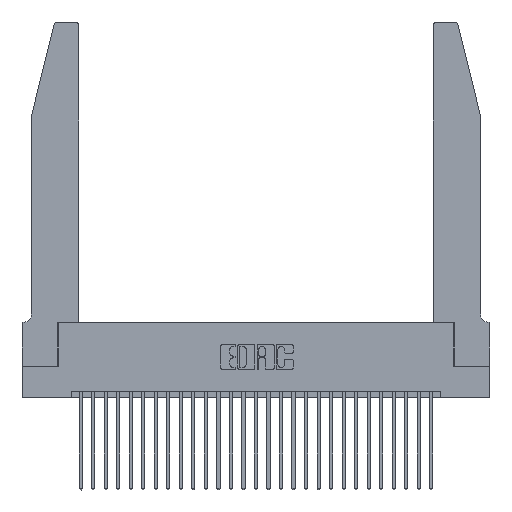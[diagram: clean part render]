
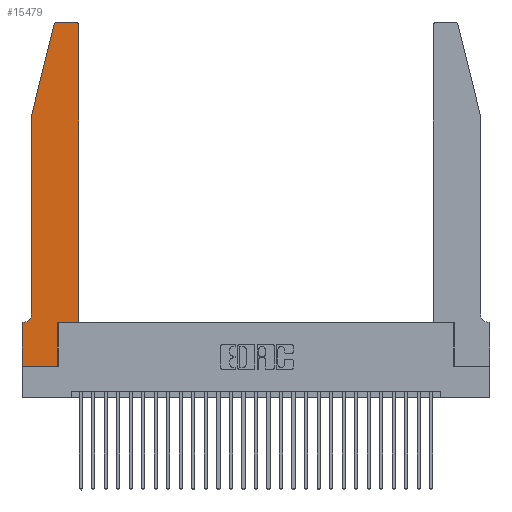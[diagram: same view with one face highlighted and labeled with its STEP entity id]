
A CAD part, top view. The second image highlights one B-rep face of the part: STEP entity #15479.
In plain terms, the highlighted planar face has unit normal (0, 0, 1).
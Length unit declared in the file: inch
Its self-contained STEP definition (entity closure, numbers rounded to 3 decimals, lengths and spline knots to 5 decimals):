
#150 = EDGE_CURVE ( 'NONE', #22027, #7102, #5964, .T. ) ;
#335 = CARTESIAN_POINT ( 'NONE',  ( 0.4505, 0.35, 0.37 ) ) ;
#549 = LINE ( 'NONE', #19431, #22512 ) ;
#706 = EDGE_CURVE ( 'NONE', #18985, #27668, #26886, .T. ) ;
#952 = ORIENTED_EDGE ( 'NONE', *, *, #706, .T. ) ;
#983 = ORIENTED_EDGE ( 'NONE', *, *, #17889, .T. ) ;
#1595 = VECTOR ( 'NONE', #10369, 39.37008 ) ;
#1600 = DIRECTION ( 'NONE',  ( 0., 0., 1. ) ) ;
#2315 = VERTEX_POINT ( 'NONE', #2986 ) ;
#2401 = EDGE_CURVE ( 'NONE', #27358, #15145, #27176, .T. ) ;
#2516 = FACE_OUTER_BOUND ( 'NONE', #24900, .T. ) ;
#2548 = DIRECTION ( 'NONE',  ( 1., 0., 0. ) ) ;
#2813 = CARTESIAN_POINT ( 'NONE',  ( 0.0055, 0.42, 0.37 ) ) ;
#2986 = CARTESIAN_POINT ( 'NONE',  ( 0.0055, 0.35, 0.37 ) ) ;
#3007 = LINE ( 'NONE', #5709, #1595 ) ;
#3257 = LINE ( 'NONE', #4641, #13493 ) ;
#3442 = CARTESIAN_POINT ( 'NONE',  ( 0.4205, 2.75, 0.37 ) ) ;
#4108 = CARTESIAN_POINT ( 'NONE',  ( 0.0755, 2., 0.37 ) ) ;
#4473 = VECTOR ( 'NONE', #17967, 39.37008 ) ;
#4641 = CARTESIAN_POINT ( 'NONE',  ( 0.2865, 0.35, 0.37 ) ) ;
#4757 = AXIS2_PLACEMENT_3D ( 'NONE', #26374, #1600, #26477 ) ;
#5021 = LINE ( 'NONE', #335, #22012 ) ;
#5185 = ORIENTED_EDGE ( 'NONE', *, *, #150, .T. ) ;
#5709 = CARTESIAN_POINT ( 'NONE',  ( 0.2605, 2.75, 0.37 ) ) ;
#5964 = LINE ( 'NONE', #22338, #27705 ) ;
#6318 = CARTESIAN_POINT ( 'NONE',  ( 0.0755, 2., 0.37 ) ) ;
#6410 = VECTOR ( 'NONE', #10379, 39.37008 ) ;
#6752 = DIRECTION ( 'NONE',  ( -0.239, -0.971, 0. ) ) ;
#7102 = VERTEX_POINT ( 'NONE', #12624 ) ;
#7559 = DIRECTION ( 'NONE',  ( 0., 1., 0. ) ) ;
#7751 = AXIS2_PLACEMENT_3D ( 'NONE', #15796, #24850, #29132 ) ;
#7936 = ORIENTED_EDGE ( 'NONE', *, *, #14590, .T. ) ;
#8402 = ORIENTED_EDGE ( 'NONE', *, *, #19738, .T. ) ;
#8673 = ORIENTED_EDGE ( 'NONE', *, *, #10531, .T. ) ;
#9144 = ORIENTED_EDGE ( 'NONE', *, *, #13209, .T. ) ;
#10369 = DIRECTION ( 'NONE',  ( -1., 0., 0. ) ) ;
#10379 = DIRECTION ( 'NONE',  ( 0., -1., 0. ) ) ;
#10531 = EDGE_CURVE ( 'NONE', #19786, #12080, #28698, .T. ) ;
#12080 = VERTEX_POINT ( 'NONE', #26515 ) ;
#12233 = LINE ( 'NONE', #22603, #4473 ) ;
#12255 = CIRCLE ( 'NONE', #23414, 0.07 ) ;
#12624 = CARTESIAN_POINT ( 'NONE',  ( 0.4505, 0.35, 0.37 ) ) ;
#12718 = DIRECTION ( 'NONE',  ( -1., 0., 0. ) ) ;
#13209 = EDGE_CURVE ( 'NONE', #12080, #2315, #12255, .T. ) ;
#13493 = VECTOR ( 'NONE', #13817, 39.37008 ) ;
#13817 = DIRECTION ( 'NONE',  ( 0., 1., 0. ) ) ;
#14590 = EDGE_CURVE ( 'NONE', #7102, #18985, #5021, .T. ) ;
#15145 = VERTEX_POINT ( 'NONE', #28821 ) ;
#15479 = ADVANCED_FACE ( 'NONE', ( #2516 ), #16470, .T. ) ;
#15796 = CARTESIAN_POINT ( 'NONE',  ( 0.4205, 2.72, 0.37 ) ) ;
#15817 = VERTEX_POINT ( 'NONE', #27545 ) ;
#16012 = CARTESIAN_POINT ( 'NONE',  ( 0.284, 2.75, 0.37 ) ) ;
#16470 = PLANE ( 'NONE',  #27087 ) ;
#17386 = VECTOR ( 'NONE', #17645, 39.37008 ) ;
#17645 = DIRECTION ( 'NONE',  ( 0., -1., 0. ) ) ;
#17889 = EDGE_CURVE ( 'NONE', #2315, #23064, #549, .T. ) ;
#17967 = DIRECTION ( 'NONE',  ( 1., 0., 0. ) ) ;
#17993 = ORIENTED_EDGE ( 'NONE', *, *, #24442, .T. ) ;
#18431 = DIRECTION ( 'NONE',  ( 0., 0., 1. ) ) ;
#18985 = VERTEX_POINT ( 'NONE', #23306 ) ;
#19431 = CARTESIAN_POINT ( 'NONE',  ( 0.0755, 0.35, 0.37 ) ) ;
#19547 = CARTESIAN_POINT ( 'NONE',  ( 0., 0., 0.37 ) ) ;
#19738 = EDGE_CURVE ( 'NONE', #27668, #27358, #3007, .T. ) ;
#19786 = VERTEX_POINT ( 'NONE', #6318 ) ;
#20870 = DIRECTION ( 'NONE',  ( 0., 0., -1. ) ) ;
#21068 = EDGE_CURVE ( 'NONE', #15817, #22027, #3257, .T. ) ;
#21802 = ORIENTED_EDGE ( 'NONE', *, *, #2401, .T. ) ;
#21895 = ORIENTED_EDGE ( 'NONE', *, *, #25765, .T. ) ;
#22012 = VECTOR ( 'NONE', #7559, 39.37008 ) ;
#22027 = VERTEX_POINT ( 'NONE', #22180 ) ;
#22100 = VECTOR ( 'NONE', #6752, 39.37008 ) ;
#22180 = CARTESIAN_POINT ( 'NONE',  ( 0.2865, 0.35, 0.37 ) ) ;
#22338 = CARTESIAN_POINT ( 'NONE',  ( 0.4505, 0.35, 0.37 ) ) ;
#22371 = CARTESIAN_POINT ( 'NONE',  ( 0., 0., 0.37 ) ) ;
#22512 = VECTOR ( 'NONE', #12718, 39.37008 ) ;
#22603 = CARTESIAN_POINT ( 'NONE',  ( 0., 0., 0.37 ) ) ;
#22789 = CARTESIAN_POINT ( 'NONE',  ( 0., 0.35, 0.37 ) ) ;
#22823 = CARTESIAN_POINT ( 'NONE',  ( 0.0755, 2., 0.37 ) ) ;
#23064 = VERTEX_POINT ( 'NONE', #26341 ) ;
#23306 = CARTESIAN_POINT ( 'NONE',  ( 0.4505, 2.72, 0.37 ) ) ;
#23414 = AXIS2_PLACEMENT_3D ( 'NONE', #2813, #20870, #25187 ) ;
#24442 = EDGE_CURVE ( 'NONE', #25166, #15817, #12233, .T. ) ;
#24499 = DIRECTION ( 'NONE',  ( 1., 0., 0. ) ) ;
#24850 = DIRECTION ( 'NONE',  ( 0., 0., 1. ) ) ;
#24900 = EDGE_LOOP ( 'NONE', ( #8402, #21802, #21895, #8673, #9144, #983, #25614, #17993, #28009, #5185, #7936, #952 ) ) ;
#25105 = LINE ( 'NONE', #19547, #6410 ) ;
#25166 = VERTEX_POINT ( 'NONE', #22371 ) ;
#25187 = DIRECTION ( 'NONE',  ( -1., 0., 0. ) ) ;
#25614 = ORIENTED_EDGE ( 'NONE', *, *, #27634, .T. ) ;
#25765 = EDGE_CURVE ( 'NONE', #15145, #19786, #27066, .T. ) ;
#26341 = CARTESIAN_POINT ( 'NONE',  ( 0., 0.35, 0.37 ) ) ;
#26374 = CARTESIAN_POINT ( 'NONE',  ( 0.284, 2.72, 0.37 ) ) ;
#26477 = DIRECTION ( 'NONE',  ( 1., 0., 0. ) ) ;
#26515 = CARTESIAN_POINT ( 'NONE',  ( 0.0755, 0.42, 0.37 ) ) ;
#26886 = CIRCLE ( 'NONE', #7751, 0.03 ) ;
#27066 = LINE ( 'NONE', #22823, #22100 ) ;
#27087 = AXIS2_PLACEMENT_3D ( 'NONE', #22789, #18431, #2548 ) ;
#27176 = CIRCLE ( 'NONE', #4757, 0.03 ) ;
#27358 = VERTEX_POINT ( 'NONE', #16012 ) ;
#27545 = CARTESIAN_POINT ( 'NONE',  ( 0.2865, 0., 0.37 ) ) ;
#27634 = EDGE_CURVE ( 'NONE', #23064, #25166, #25105, .T. ) ;
#27668 = VERTEX_POINT ( 'NONE', #3442 ) ;
#27705 = VECTOR ( 'NONE', #24499, 39.37008 ) ;
#28009 = ORIENTED_EDGE ( 'NONE', *, *, #21068, .T. ) ;
#28698 = LINE ( 'NONE', #4108, #17386 ) ;
#28821 = CARTESIAN_POINT ( 'NONE',  ( 0.25487, 2.72718, 0.37 ) ) ;
#29132 = DIRECTION ( 'NONE',  ( 1., 0., 0. ) ) ;
